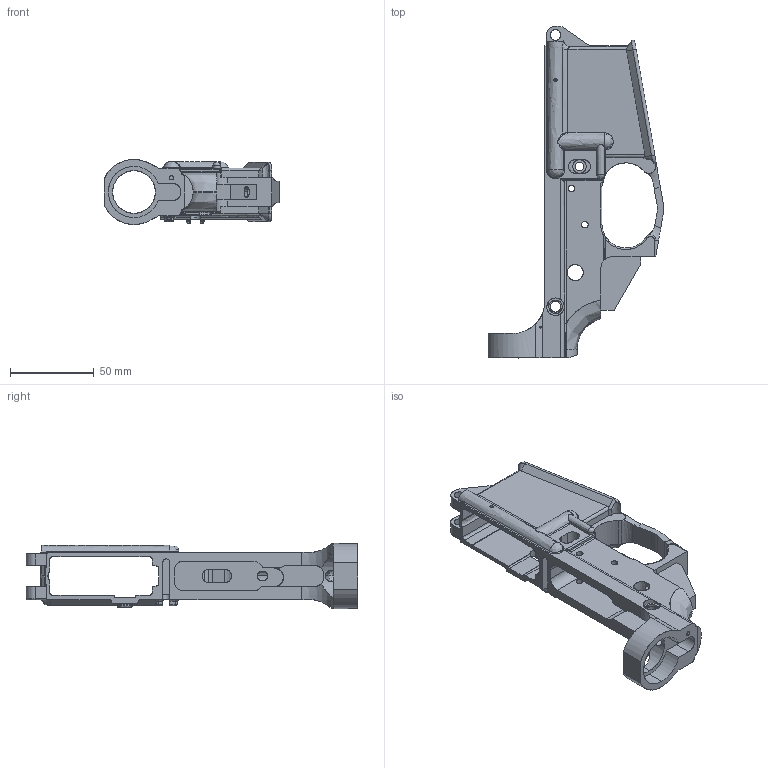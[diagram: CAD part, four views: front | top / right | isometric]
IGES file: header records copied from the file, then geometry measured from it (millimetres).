
Start section: SolidWorks IGES file using analytic representation for surfaces
Global section: file name: MKIIb reciever.IGS; native system: SolidWorks 2012; preprocessor: SolidWorks 2012; author: Pld; date: 130926.052202; units: inch
Bounding box: 104.43 x 197.71 x 38.74 mm (x, y, z)
Surface area: 55156.3 mm2 (no closed solid volume)
Topology: 0 solids, 0 shells, 531 faces, 7399 edges, 7378 vertices
Faces by surface type: bspline 278, revolution 253
